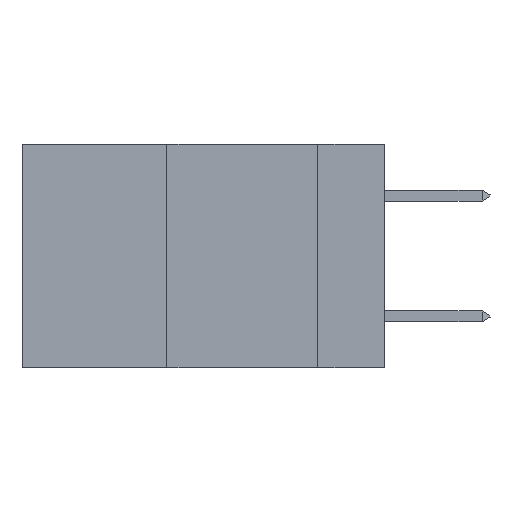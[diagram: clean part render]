
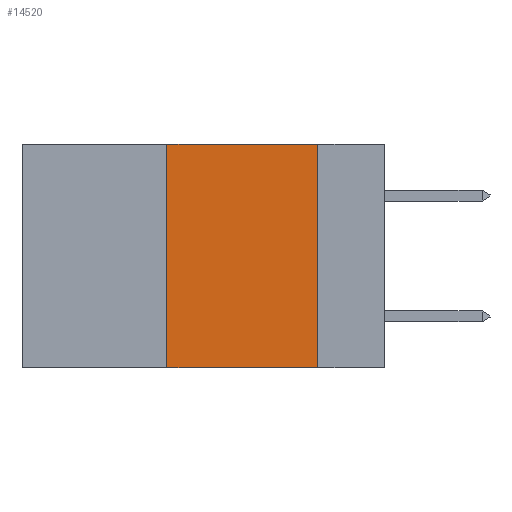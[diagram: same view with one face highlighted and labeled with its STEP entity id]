
A CAD part, left-side view. The second image highlights one B-rep face of the part: STEP entity #14520.
In plain terms, the highlighted planar face has unit normal (-1, 0, 0).
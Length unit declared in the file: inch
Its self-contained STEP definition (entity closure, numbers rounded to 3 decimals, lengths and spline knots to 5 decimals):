
#510 = CARTESIAN_POINT ( 'NONE',  ( 0., 0.6, -0.37 ) ) ;
#1122 = ORIENTED_EDGE ( 'NONE', *, *, #6057, .F. ) ;
#1405 = DIRECTION ( 'NONE',  ( 0., 0., -1. ) ) ;
#2030 = ORIENTED_EDGE ( 'NONE', *, *, #4437, .F. ) ;
#3160 = ORIENTED_EDGE ( 'NONE', *, *, #7859, .F. ) ;
#4206 = CARTESIAN_POINT ( 'NONE',  ( 0., 0.36, -0.37 ) ) ;
#4437 = EDGE_CURVE ( 'NONE', #7928, #30559, #14297, .T. ) ;
#6057 = EDGE_CURVE ( 'NONE', #30559, #7801, #13936, .T. ) ;
#7022 = PLANE ( 'NONE',  #21136 ) ;
#7496 = CARTESIAN_POINT ( 'NONE',  ( 0., 0.36, 0. ) ) ;
#7801 = VERTEX_POINT ( 'NONE', #10934 ) ;
#7859 = EDGE_CURVE ( 'NONE', #7801, #18659, #8285, .T. ) ;
#7928 = VERTEX_POINT ( 'NONE', #4206 ) ;
#8285 = LINE ( 'NONE', #18128, #19352 ) ;
#10934 = CARTESIAN_POINT ( 'NONE',  ( 0., 0.11, 0. ) ) ;
#12259 = EDGE_CURVE ( 'NONE', #7928, #18659, #27249, .T. ) ;
#13190 = VECTOR ( 'NONE', #13897, 39.37008 ) ;
#13897 = DIRECTION ( 'NONE',  ( 0., -1., 0. ) ) ;
#13936 = LINE ( 'NONE', #25535, #13190 ) ;
#14160 = CARTESIAN_POINT ( 'NONE',  ( 0., 0.6, 0. ) ) ;
#14297 = LINE ( 'NONE', #7496, #25983 ) ;
#14520 = ADVANCED_FACE ( 'NONE', ( #18437 ), #7022, .F. ) ;
#16531 = DIRECTION ( 'NONE',  ( 0., 0., -1. ) ) ;
#16716 = ORIENTED_EDGE ( 'NONE', *, *, #12259, .T. ) ;
#17257 = DIRECTION ( 'NONE',  ( 0., -1., 0. ) ) ;
#18128 = CARTESIAN_POINT ( 'NONE',  ( 0., 0.11, 0. ) ) ;
#18437 = FACE_OUTER_BOUND ( 'NONE', #24690, .T. ) ;
#18659 = VERTEX_POINT ( 'NONE', #26133 ) ;
#19352 = VECTOR ( 'NONE', #1405, 39.37008 ) ;
#21136 = AXIS2_PLACEMENT_3D ( 'NONE', #14160, #30463, #16531 ) ;
#22540 = CARTESIAN_POINT ( 'NONE',  ( 0., 0.36, 0. ) ) ;
#24227 = DIRECTION ( 'NONE',  ( 0., 0., 1. ) ) ;
#24690 = EDGE_LOOP ( 'NONE', ( #3160, #1122, #2030, #16716 ) ) ;
#25535 = CARTESIAN_POINT ( 'NONE',  ( 0., 0.6, 0. ) ) ;
#25983 = VECTOR ( 'NONE', #24227, 39.37008 ) ;
#26133 = CARTESIAN_POINT ( 'NONE',  ( 0., 0.11, -0.37 ) ) ;
#26515 = VECTOR ( 'NONE', #17257, 39.37008 ) ;
#27249 = LINE ( 'NONE', #510, #26515 ) ;
#30463 = DIRECTION ( 'NONE',  ( 1., 0., 0. ) ) ;
#30559 = VERTEX_POINT ( 'NONE', #22540 ) ;
